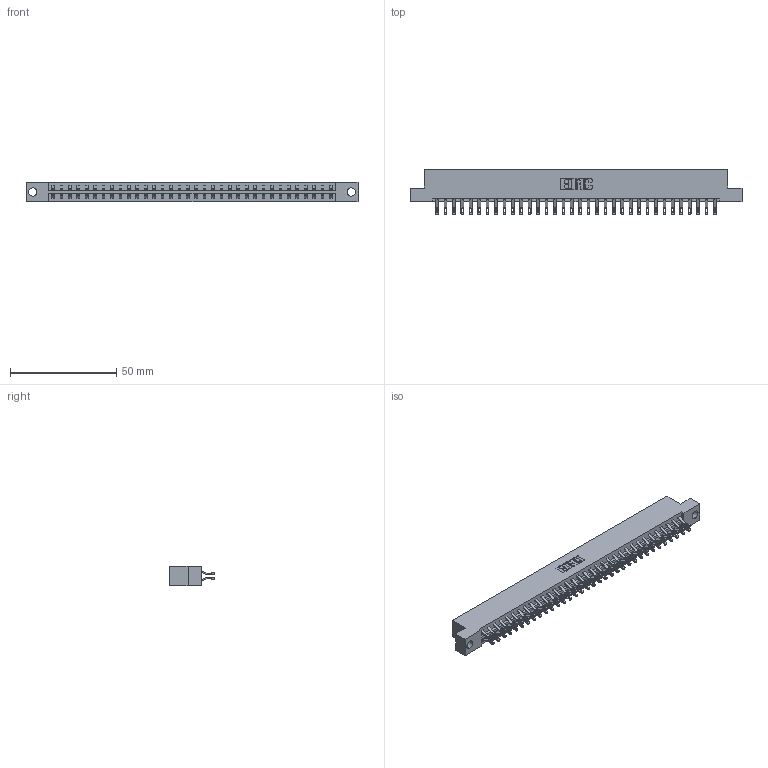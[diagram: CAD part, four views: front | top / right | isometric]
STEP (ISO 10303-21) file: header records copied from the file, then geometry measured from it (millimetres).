
FILE_DESCRIPTION (( 'STEP AP203' ), '1' );
FILE_NAME ('833-068-555-204.STEP', '2020-06-05T11:04:31', ( '' ), ( '' ), 'SwSTEP 2.0', 'SolidWorks 2020', '' );
FILE_SCHEMA (( 'CONFIG_CONTROL_DESIGN' ));
Length unit declared in the file: inch
Products named in the file (3): 833 Part_Flush - .156 Dia - TH; 833-068-555-204; 345-292-001_555 Tail
Assembly tree (69 placements, depth 2):
  833-068-555-204
    833 Part_Flush - .156 Dia - TH
    345-292-001_555 Tail  x68
Bounding box: 156.26 x 21.47 x 9.4 mm (x, y, z)
Volume: 15987.9 mm3; surface area: 19352.8 mm2
Topology: 69 solids, 69 shells, 4058 faces, 12755 edges, 8502 vertices
Faces by surface type: plane 2382, cylinder 1676
Entity records: 23237 total; most frequent: CARTESIAN_POINT 3896, ORIENTED_EDGE 3802, DIRECTION 3313, EDGE_CURVE 1901, LINE 1753, VECTOR 1753, VERTEX_POINT 1266, AXIS2_PLACEMENT_3D 780
